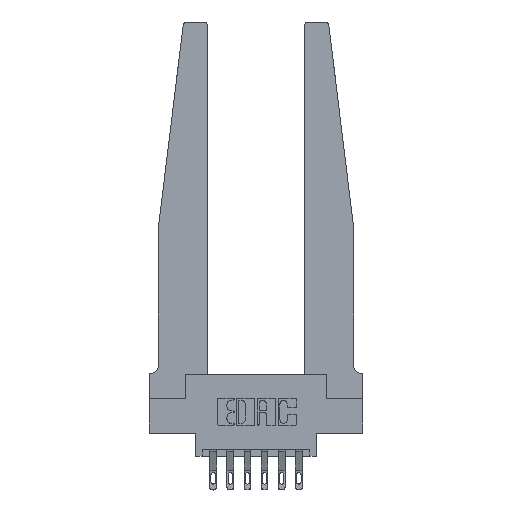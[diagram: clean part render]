
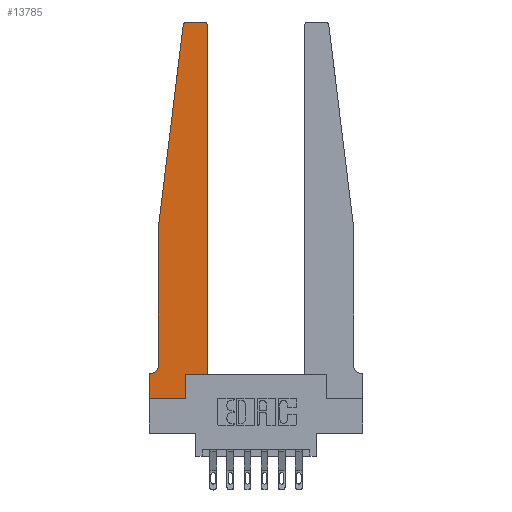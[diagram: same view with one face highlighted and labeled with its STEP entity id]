
A CAD part, top view. The second image highlights one B-rep face of the part: STEP entity #13785.
In plain terms, the highlighted planar face has unit normal (0, 0, 1).
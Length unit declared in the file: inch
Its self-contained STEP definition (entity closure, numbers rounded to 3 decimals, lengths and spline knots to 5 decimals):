
#58 = ORIENTED_EDGE ( 'NONE', *, *, #10096, .T. ) ;
#206 = VERTEX_POINT ( 'NONE', #7634 ) ;
#228 = DIRECTION ( 'NONE',  ( 0., -1., 0. ) ) ;
#246 = VECTOR ( 'NONE', #10108, 39.37008 ) ;
#352 = EDGE_CURVE ( 'NONE', #541, #6536, #2143, .T. ) ;
#407 = CARTESIAN_POINT ( 'NONE',  ( 0.24675, 2.72367, 0.37 ) ) ;
#446 = CARTESIAN_POINT ( 'NONE',  ( 0.065, 1.25, 0.37 ) ) ;
#495 = CARTESIAN_POINT ( 'NONE',  ( 0.425, 0.18, 0.37 ) ) ;
#518 = CARTESIAN_POINT ( 'NONE',  ( 0., 0.1875, 0.37 ) ) ;
#522 = DIRECTION ( 'NONE',  ( 1., 0., 0. ) ) ;
#541 = VERTEX_POINT ( 'NONE', #518 ) ;
#554 = DIRECTION ( 'NONE',  ( 1., 0., 0. ) ) ;
#584 = EDGE_CURVE ( 'NONE', #4421, #2374, #10906, .T. ) ;
#1010 = ORIENTED_EDGE ( 'NONE', *, *, #5930, .T. ) ;
#1016 = ORIENTED_EDGE ( 'NONE', *, *, #2427, .T. ) ;
#1160 = CARTESIAN_POINT ( 'NONE',  ( 0.425, 0.18, 0.37 ) ) ;
#1178 = DIRECTION ( 'NONE',  ( 1., 0., 0. ) ) ;
#1230 = DIRECTION ( 'NONE',  ( -1., 0., 0. ) ) ;
#1277 = VECTOR ( 'NONE', #1571, 39.37008 ) ;
#1283 = AXIS2_PLACEMENT_3D ( 'NONE', #2088, #9678, #3188 ) ;
#1571 = DIRECTION ( 'NONE',  ( 0., 1., 0. ) ) ;
#1620 = LINE ( 'NONE', #7748, #10588 ) ;
#1935 = CARTESIAN_POINT ( 'NONE',  ( 0., 0., 0.37 ) ) ;
#1948 = LINE ( 'NONE', #446, #10570 ) ;
#2088 = CARTESIAN_POINT ( 'NONE',  ( 0., 0.1875, 0.37 ) ) ;
#2132 = EDGE_CURVE ( 'NONE', #3583, #2452, #10410, .T. ) ;
#2143 = LINE ( 'NONE', #1935, #5048 ) ;
#2374 = VERTEX_POINT ( 'NONE', #1160 ) ;
#2427 = EDGE_CURVE ( 'NONE', #5269, #8341, #1948, .T. ) ;
#2452 = VERTEX_POINT ( 'NONE', #10488 ) ;
#2661 = ORIENTED_EDGE ( 'NONE', *, *, #3133, .T. ) ;
#2956 = AXIS2_PLACEMENT_3D ( 'NONE', #13510, #7051, #554 ) ;
#2987 = CARTESIAN_POINT ( 'NONE',  ( 0.395, 2.75, 0.37 ) ) ;
#3128 = LINE ( 'NONE', #11163, #246 ) ;
#3133 = EDGE_CURVE ( 'NONE', #8341, #6498, #3630, .T. ) ;
#3188 = DIRECTION ( 'NONE',  ( 1., 0., 0. ) ) ;
#3191 = DIRECTION ( 'NONE',  ( 0., 0., -1. ) ) ;
#3277 = DIRECTION ( 'NONE',  ( 1., 0., 0. ) ) ;
#3583 = VERTEX_POINT ( 'NONE', #2987 ) ;
#3630 = CIRCLE ( 'NONE', #7541, 0.05 ) ;
#3633 = ORIENTED_EDGE ( 'NONE', *, *, #11447, .T. ) ;
#3773 = CARTESIAN_POINT ( 'NONE',  ( 0., 0., 0.37 ) ) ;
#3997 = LINE ( 'NONE', #5070, #6507 ) ;
#4030 = VERTEX_POINT ( 'NONE', #11216 ) ;
#4079 = CARTESIAN_POINT ( 'NONE',  ( 0.065, 0.2375, 0.37 ) ) ;
#4409 = VERTEX_POINT ( 'NONE', #407 ) ;
#4421 = VERTEX_POINT ( 'NONE', #13417 ) ;
#4555 = DIRECTION ( 'NONE',  ( 0., -1., 0. ) ) ;
#4914 = DIRECTION ( 'NONE',  ( -1., 0., 0. ) ) ;
#4993 = CARTESIAN_POINT ( 'NONE',  ( 0.25, 2.75, 0.37 ) ) ;
#5048 = VECTOR ( 'NONE', #4555, 39.37008 ) ;
#5070 = CARTESIAN_POINT ( 'NONE',  ( 0.2605, 0.18, 0.37 ) ) ;
#5269 = VERTEX_POINT ( 'NONE', #13338 ) ;
#5525 = LINE ( 'NONE', #10815, #13476 ) ;
#5874 = VECTOR ( 'NONE', #1178, 39.37008 ) ;
#5930 = EDGE_CURVE ( 'NONE', #2452, #4409, #13178, .T. ) ;
#6498 = VERTEX_POINT ( 'NONE', #12282 ) ;
#6507 = VECTOR ( 'NONE', #12601, 39.37008 ) ;
#6536 = VERTEX_POINT ( 'NONE', #3773 ) ;
#7014 = DIRECTION ( 'NONE',  ( 0., 0., 1. ) ) ;
#7051 = DIRECTION ( 'NONE',  ( 0., 0., 1. ) ) ;
#7165 = EDGE_CURVE ( 'NONE', #4030, #3583, #12963, .T. ) ;
#7493 = PLANE ( 'NONE',  #1283 ) ;
#7541 = AXIS2_PLACEMENT_3D ( 'NONE', #9684, #3191, #10726 ) ;
#7634 = CARTESIAN_POINT ( 'NONE',  ( 0.2605, 0., 0.37 ) ) ;
#7748 = CARTESIAN_POINT ( 'NONE',  ( 0.065, 0.1875, 0.37 ) ) ;
#8341 = VERTEX_POINT ( 'NONE', #4079 ) ;
#8803 = EDGE_CURVE ( 'NONE', #2374, #4030, #9925, .T. ) ;
#8903 = ORIENTED_EDGE ( 'NONE', *, *, #2132, .T. ) ;
#9228 = ORIENTED_EDGE ( 'NONE', *, *, #584, .T. ) ;
#9366 = ORIENTED_EDGE ( 'NONE', *, *, #8803, .T. ) ;
#9678 = DIRECTION ( 'NONE',  ( 0., 0., 1. ) ) ;
#9684 = CARTESIAN_POINT ( 'NONE',  ( 0.015, 0.2375, 0.37 ) ) ;
#9899 = EDGE_CURVE ( 'NONE', #4409, #5269, #3128, .T. ) ;
#9925 = LINE ( 'NONE', #495, #1277 ) ;
#10037 = FACE_OUTER_BOUND ( 'NONE', #12080, .T. ) ;
#10096 = EDGE_CURVE ( 'NONE', #206, #4421, #3997, .T. ) ;
#10108 = DIRECTION ( 'NONE',  ( -0.122, -0.992, 0. ) ) ;
#10410 = LINE ( 'NONE', #4993, #11052 ) ;
#10488 = CARTESIAN_POINT ( 'NONE',  ( 0.27653, 2.75, 0.37 ) ) ;
#10570 = VECTOR ( 'NONE', #228, 39.37008 ) ;
#10588 = VECTOR ( 'NONE', #1230, 39.37008 ) ;
#10726 = DIRECTION ( 'NONE',  ( -1., 0., 0. ) ) ;
#10815 = CARTESIAN_POINT ( 'NONE',  ( 0., 0., 0.37 ) ) ;
#10906 = LINE ( 'NONE', #11893, #5874 ) ;
#11052 = VECTOR ( 'NONE', #4914, 39.37008 ) ;
#11163 = CARTESIAN_POINT ( 'NONE',  ( 0.065, 1.25, 0.37 ) ) ;
#11216 = CARTESIAN_POINT ( 'NONE',  ( 0.425, 2.72, 0.37 ) ) ;
#11376 = EDGE_CURVE ( 'NONE', #6536, #206, #5525, .T. ) ;
#11447 = EDGE_CURVE ( 'NONE', #6498, #541, #1620, .T. ) ;
#11893 = CARTESIAN_POINT ( 'NONE',  ( 0.425, 0.18, 0.37 ) ) ;
#12080 = EDGE_LOOP ( 'NONE', ( #8903, #1010, #13291, #1016, #2661, #3633, #12592, #13411, #58, #9228, #9366, #13572 ) ) ;
#12282 = CARTESIAN_POINT ( 'NONE',  ( 0.015, 0.1875, 0.37 ) ) ;
#12592 = ORIENTED_EDGE ( 'NONE', *, *, #352, .T. ) ;
#12601 = DIRECTION ( 'NONE',  ( 0., 1., 0. ) ) ;
#12963 = CIRCLE ( 'NONE', #13742, 0.03 ) ;
#13178 = CIRCLE ( 'NONE', #2956, 0.03 ) ;
#13291 = ORIENTED_EDGE ( 'NONE', *, *, #9899, .T. ) ;
#13338 = CARTESIAN_POINT ( 'NONE',  ( 0.065, 1.25, 0.37 ) ) ;
#13411 = ORIENTED_EDGE ( 'NONE', *, *, #11376, .T. ) ;
#13417 = CARTESIAN_POINT ( 'NONE',  ( 0.2605, 0.18, 0.37 ) ) ;
#13476 = VECTOR ( 'NONE', #3277, 39.37008 ) ;
#13478 = CARTESIAN_POINT ( 'NONE',  ( 0.395, 2.72, 0.37 ) ) ;
#13510 = CARTESIAN_POINT ( 'NONE',  ( 0.27653, 2.72, 0.37 ) ) ;
#13572 = ORIENTED_EDGE ( 'NONE', *, *, #7165, .T. ) ;
#13742 = AXIS2_PLACEMENT_3D ( 'NONE', #13478, #7014, #522 ) ;
#13785 = ADVANCED_FACE ( 'NONE', ( #10037 ), #7493, .T. ) ;
